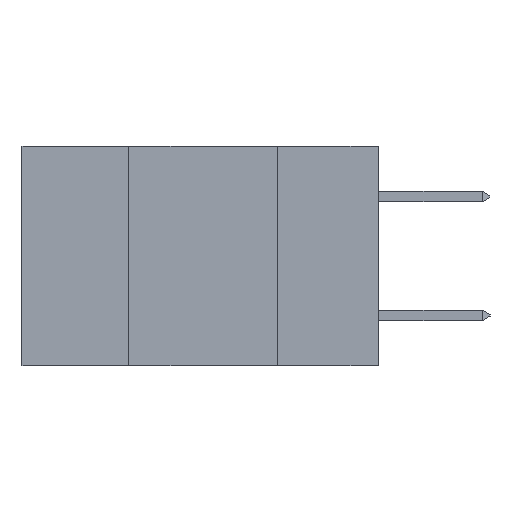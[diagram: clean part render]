
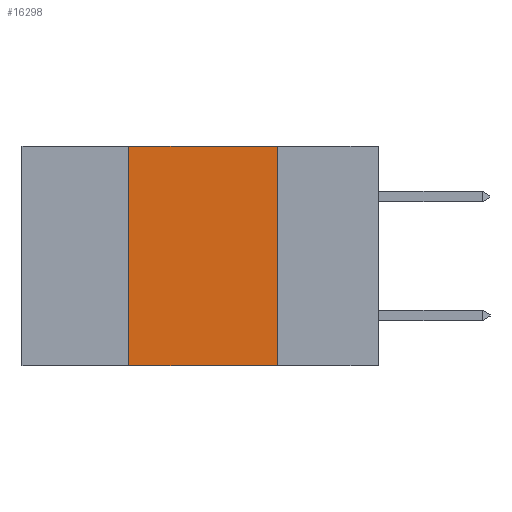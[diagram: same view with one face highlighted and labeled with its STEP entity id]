
A CAD part, left-side view. The second image highlights one B-rep face of the part: STEP entity #16298.
In plain terms, the highlighted planar face has unit normal (-1, 0, 0).
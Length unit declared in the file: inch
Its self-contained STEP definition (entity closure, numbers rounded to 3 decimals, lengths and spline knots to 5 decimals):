
#396 = PLANE ( 'NONE',  #7143 ) ;
#949 = CARTESIAN_POINT ( 'NONE',  ( 0., 0.17, -0.37 ) ) ;
#1490 = LINE ( 'NONE', #8320, #2148 ) ;
#2102 = DIRECTION ( 'NONE',  ( 0., -1., 0. ) ) ;
#2148 = VECTOR ( 'NONE', #2102, 39.37008 ) ;
#2480 = DIRECTION ( 'NONE',  ( 1., 0., 0. ) ) ;
#3108 = VERTEX_POINT ( 'NONE', #4917 ) ;
#3696 = CARTESIAN_POINT ( 'NONE',  ( 0., 0.6, 0. ) ) ;
#4049 = VERTEX_POINT ( 'NONE', #9752 ) ;
#4917 = CARTESIAN_POINT ( 'NONE',  ( 0., 0.42, -0.37 ) ) ;
#6233 = CARTESIAN_POINT ( 'NONE',  ( 0., 0.17, -0.37 ) ) ;
#6671 = ORIENTED_EDGE ( 'NONE', *, *, #13978, .T. ) ;
#7143 = AXIS2_PLACEMENT_3D ( 'NONE', #12706, #2480, #16770 ) ;
#7210 = FACE_OUTER_BOUND ( 'NONE', #16680, .T. ) ;
#7984 = ORIENTED_EDGE ( 'NONE', *, *, #16523, .F. ) ;
#8174 = VECTOR ( 'NONE', #17335, 39.37008 ) ;
#8310 = ORIENTED_EDGE ( 'NONE', *, *, #15679, .F. ) ;
#8320 = CARTESIAN_POINT ( 'NONE',  ( 0., 0.6, -0.37 ) ) ;
#9752 = CARTESIAN_POINT ( 'NONE',  ( 0., 0.42, 0. ) ) ;
#12706 = CARTESIAN_POINT ( 'NONE',  ( 0., 0.6, 0. ) ) ;
#13428 = ORIENTED_EDGE ( 'NONE', *, *, #13804, .F. ) ;
#13804 = EDGE_CURVE ( 'NONE', #4049, #22244, #16270, .T. ) ;
#13978 = EDGE_CURVE ( 'NONE', #3108, #18881, #1490, .T. ) ;
#15679 = EDGE_CURVE ( 'NONE', #22244, #18881, #24306, .T. ) ;
#16270 = LINE ( 'NONE', #3696, #20981 ) ;
#16298 = ADVANCED_FACE ( 'NONE', ( #7210 ), #396, .F. ) ;
#16523 = EDGE_CURVE ( 'NONE', #3108, #4049, #23065, .T. ) ;
#16680 = EDGE_LOOP ( 'NONE', ( #8310, #13428, #7984, #6671 ) ) ;
#16770 = DIRECTION ( 'NONE',  ( 0., 0., -1. ) ) ;
#17335 = DIRECTION ( 'NONE',  ( 0., 0., -1. ) ) ;
#17714 = VECTOR ( 'NONE', #19396, 39.37008 ) ;
#18881 = VERTEX_POINT ( 'NONE', #6233 ) ;
#19396 = DIRECTION ( 'NONE',  ( 0., 0., 1. ) ) ;
#20981 = VECTOR ( 'NONE', #23983, 39.37008 ) ;
#21336 = CARTESIAN_POINT ( 'NONE',  ( 0., 0.42, -0.37 ) ) ;
#22244 = VERTEX_POINT ( 'NONE', #23637 ) ;
#23065 = LINE ( 'NONE', #21336, #17714 ) ;
#23637 = CARTESIAN_POINT ( 'NONE',  ( 0., 0.17, 0. ) ) ;
#23983 = DIRECTION ( 'NONE',  ( 0., -1., 0. ) ) ;
#24306 = LINE ( 'NONE', #949, #8174 ) ;
